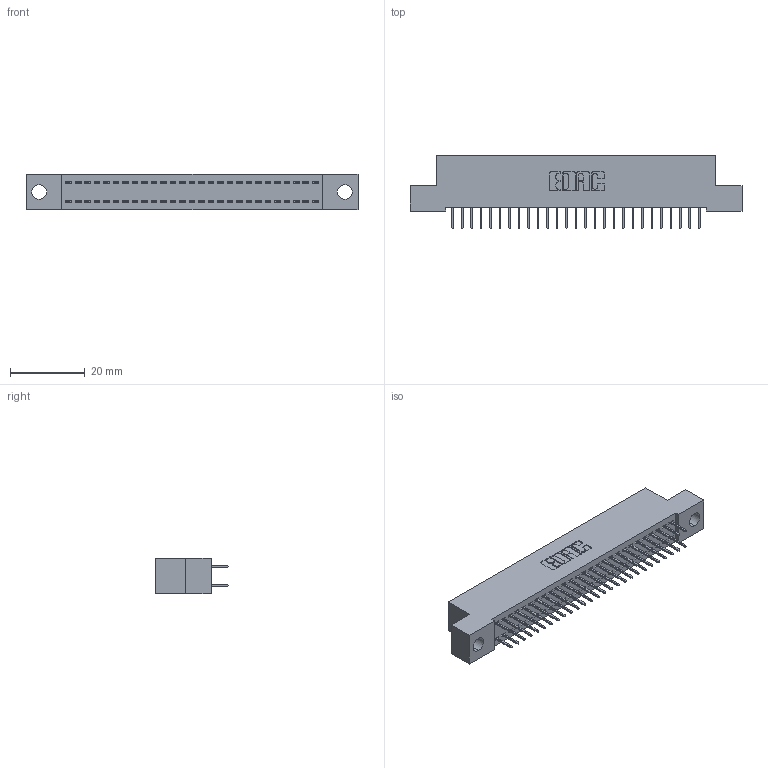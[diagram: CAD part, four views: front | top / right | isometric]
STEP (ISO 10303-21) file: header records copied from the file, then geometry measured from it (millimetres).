
FILE_DESCRIPTION (( 'STEP AP203' ), '1' );
FILE_NAME ('342-054-524-204.STEP', '2019-10-03T03:01:35', ( '' ), ( '' ), 'SwSTEP 2.0', 'SolidWorks 2016', '' );
FILE_SCHEMA (( 'CONFIG_CONTROL_DESIGN' ));
Length unit declared in the file: inch
Products named in the file (3): 342 Part_.156 TH; 345-292-001_345-293-124; 342-054-524-204
Assembly tree (55 placements, depth 2):
  342-054-524-204
    342 Part_.156 TH
    345-292-001_345-293-124  x54
Bounding box: 88.9 x 19.69 x 9.4 mm (x, y, z)
Volume: 7747.9 mm3; surface area: 11853.7 mm2
Topology: 55 solids, 55 shells, 3134 faces, 8885 edges, 5706 vertices
Faces by surface type: plane 2334, cylinder 800
Entity records: 19255 total; most frequent: CARTESIAN_POINT 3206, ORIENTED_EDGE 3142, DIRECTION 2767, EDGE_CURVE 1571, LINE 1447, VECTOR 1447, VERTEX_POINT 1042, AXIS2_PLACEMENT_3D 660
